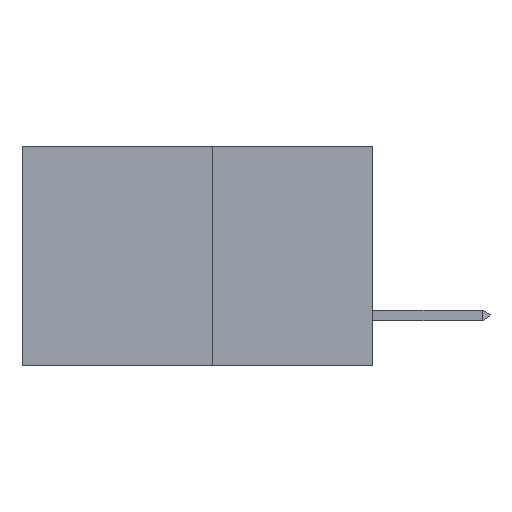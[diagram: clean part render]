
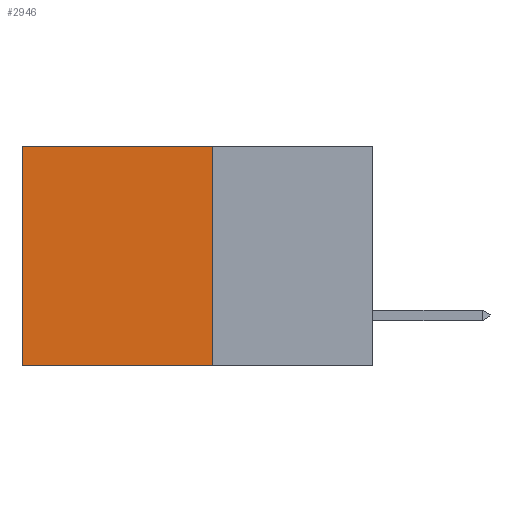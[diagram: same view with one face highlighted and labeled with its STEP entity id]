
A CAD part, left-side view. The second image highlights one B-rep face of the part: STEP entity #2946.
In plain terms, the highlighted planar face has unit normal (-1, 0, 0).
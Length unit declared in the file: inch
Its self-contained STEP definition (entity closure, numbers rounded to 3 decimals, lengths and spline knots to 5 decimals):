
#309 = CARTESIAN_POINT ( 'NONE',  ( 0.277, 0.27, -0.37 ) ) ;
#455 = CARTESIAN_POINT ( 'NONE',  ( 0.277, 0.59, 0. ) ) ;
#862 = LINE ( 'NONE', #309, #3395 ) ;
#1080 = DIRECTION ( 'NONE',  ( 0., 0., -1. ) ) ;
#1123 = EDGE_LOOP ( 'NONE', ( #8141, #8458, #9100, #1277 ) ) ;
#1131 = CARTESIAN_POINT ( 'NONE',  ( 0.277, 0.59, -0.37 ) ) ;
#1277 = ORIENTED_EDGE ( 'NONE', *, *, #11151, .T. ) ;
#1344 = CARTESIAN_POINT ( 'NONE',  ( 0.277, 0.27, -0.37 ) ) ;
#1577 = FACE_OUTER_BOUND ( 'NONE', #1123, .T. ) ;
#1710 = VERTEX_POINT ( 'NONE', #455 ) ;
#2290 = CARTESIAN_POINT ( 'NONE',  ( 0.277, 0.27, -0.37 ) ) ;
#2450 = LINE ( 'NONE', #1131, #7791 ) ;
#2888 = VECTOR ( 'NONE', #9663, 39.37008 ) ;
#2946 = ADVANCED_FACE ( 'NONE', ( #1577 ), #12205, .F. ) ;
#3395 = VECTOR ( 'NONE', #12936, 39.37008 ) ;
#3440 = EDGE_CURVE ( 'NONE', #10803, #11813, #862, .T. ) ;
#4828 = EDGE_CURVE ( 'NONE', #11813, #13001, #10559, .T. ) ;
#4837 = CARTESIAN_POINT ( 'NONE',  ( 0.277, 0.59, -0.37 ) ) ;
#4897 = CARTESIAN_POINT ( 'NONE',  ( 0.277, 0.27, 0. ) ) ;
#5253 = EDGE_CURVE ( 'NONE', #1710, #13001, #2450, .T. ) ;
#5743 = LINE ( 'NONE', #11767, #2888 ) ;
#7791 = VECTOR ( 'NONE', #1080, 39.37008 ) ;
#8141 = ORIENTED_EDGE ( 'NONE', *, *, #5253, .T. ) ;
#8458 = ORIENTED_EDGE ( 'NONE', *, *, #4828, .F. ) ;
#8880 = CARTESIAN_POINT ( 'NONE',  ( 0.277, 0.27, -0.37 ) ) ;
#8996 = DIRECTION ( 'NONE',  ( 0., 1., 0. ) ) ;
#9100 = ORIENTED_EDGE ( 'NONE', *, *, #3440, .F. ) ;
#9327 = AXIS2_PLACEMENT_3D ( 'NONE', #1344, #10004, #11914 ) ;
#9663 = DIRECTION ( 'NONE',  ( 0., 1., 0. ) ) ;
#10004 = DIRECTION ( 'NONE',  ( 1., 0., 0. ) ) ;
#10226 = VECTOR ( 'NONE', #8996, 39.37008 ) ;
#10559 = LINE ( 'NONE', #8880, #10226 ) ;
#10803 = VERTEX_POINT ( 'NONE', #4897 ) ;
#11151 = EDGE_CURVE ( 'NONE', #10803, #1710, #5743, .T. ) ;
#11767 = CARTESIAN_POINT ( 'NONE',  ( 0.277, 0.27, 0. ) ) ;
#11813 = VERTEX_POINT ( 'NONE', #2290 ) ;
#11914 = DIRECTION ( 'NONE',  ( 0., 0., -1. ) ) ;
#12205 = PLANE ( 'NONE',  #9327 ) ;
#12936 = DIRECTION ( 'NONE',  ( 0., 0., -1. ) ) ;
#13001 = VERTEX_POINT ( 'NONE', #4837 ) ;
